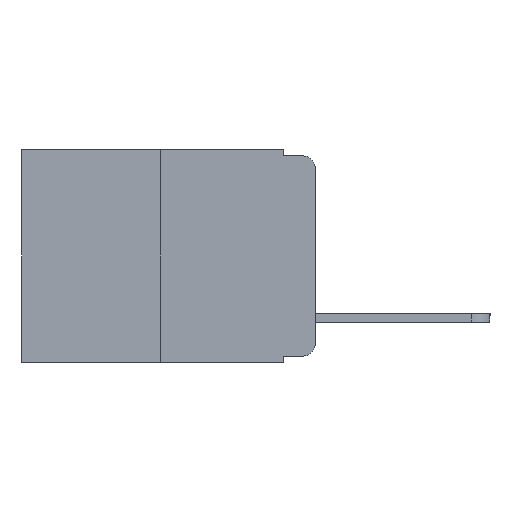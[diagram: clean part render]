
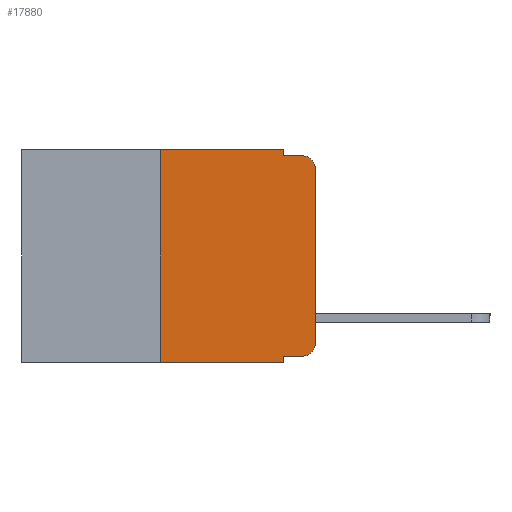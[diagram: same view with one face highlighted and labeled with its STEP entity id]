
A CAD part, left-side view. The second image highlights one B-rep face of the part: STEP entity #17880.
In plain terms, the highlighted planar face has unit normal (-1, 0, 0).
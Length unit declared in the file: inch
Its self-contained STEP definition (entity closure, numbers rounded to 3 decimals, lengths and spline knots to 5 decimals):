
#345 = EDGE_CURVE ( 'NONE', #1542, #9815, #5355, .T. ) ;
#1218 = CARTESIAN_POINT ( 'NONE',  ( 0., 0.02, -0.03 ) ) ;
#1253 = VECTOR ( 'NONE', #8142, 39.37008 ) ;
#1542 = VERTEX_POINT ( 'NONE', #8041 ) ;
#1605 = LINE ( 'NONE', #11146, #16350 ) ;
#2060 = CARTESIAN_POINT ( 'NONE',  ( 0., 0.051, 0. ) ) ;
#2106 = AXIS2_PLACEMENT_3D ( 'NONE', #1218, #11420, #2782 ) ;
#2268 = ORIENTED_EDGE ( 'NONE', *, *, #15276, .F. ) ;
#2299 = DIRECTION ( 'NONE',  ( 1., 0., 0. ) ) ;
#2311 = ORIENTED_EDGE ( 'NONE', *, *, #17517, .F. ) ;
#2459 = ORIENTED_EDGE ( 'NONE', *, *, #16205, .F. ) ;
#2679 = VECTOR ( 'NONE', #14028, 39.37008 ) ;
#2782 = DIRECTION ( 'NONE',  ( 0., 0., -1. ) ) ;
#2800 = ORIENTED_EDGE ( 'NONE', *, *, #17160, .F. ) ;
#2856 = CARTESIAN_POINT ( 'NONE',  ( 0., 0.051, -0.343 ) ) ;
#3518 = VECTOR ( 'NONE', #6257, 39.37008 ) ;
#3520 = VERTEX_POINT ( 'NONE', #3736 ) ;
#3658 = DIRECTION ( 'NONE',  ( 0., 0., -1. ) ) ;
#3736 = CARTESIAN_POINT ( 'NONE',  ( 0., 0.02, -0.01 ) ) ;
#4001 = CARTESIAN_POINT ( 'NONE',  ( 0., 0., 0. ) ) ;
#4339 = VERTEX_POINT ( 'NONE', #2856 ) ;
#4696 = AXIS2_PLACEMENT_3D ( 'NONE', #4937, #14725, #6358 ) ;
#4819 = CARTESIAN_POINT ( 'NONE',  ( 0., 0.25, 0. ) ) ;
#4910 = VECTOR ( 'NONE', #3658, 39.37008 ) ;
#4937 = CARTESIAN_POINT ( 'NONE',  ( 0., 0.02, -0.313 ) ) ;
#5074 = EDGE_LOOP ( 'NONE', ( #12669, #11623, #2800, #2459, #2311, #2268, #10667, #10511, #12202, #16881 ) ) ;
#5111 = CARTESIAN_POINT ( 'NONE',  ( 0., 0.473, -0.343 ) ) ;
#5220 = LINE ( 'NONE', #5350, #12689 ) ;
#5350 = CARTESIAN_POINT ( 'NONE',  ( 0., 0.051, -0.333 ) ) ;
#5355 = LINE ( 'NONE', #4001, #1253 ) ;
#5540 = LINE ( 'NONE', #14225, #15814 ) ;
#5560 = EDGE_CURVE ( 'NONE', #10413, #4339, #9112, .T. ) ;
#6257 = DIRECTION ( 'NONE',  ( 0., 0., 1. ) ) ;
#6358 = DIRECTION ( 'NONE',  ( 0., 0., -1. ) ) ;
#7493 = AXIS2_PLACEMENT_3D ( 'NONE', #7959, #2299, #12383 ) ;
#7753 = CARTESIAN_POINT ( 'NONE',  ( 0., 0.25, -0.343 ) ) ;
#7959 = CARTESIAN_POINT ( 'NONE',  ( 0., 0.473, 0. ) ) ;
#8041 = CARTESIAN_POINT ( 'NONE',  ( 0., 0., -0.313 ) ) ;
#8142 = DIRECTION ( 'NONE',  ( 0., 0., 1. ) ) ;
#8289 = CARTESIAN_POINT ( 'NONE',  ( 0., 0.02, -0.333 ) ) ;
#9112 = LINE ( 'NONE', #5111, #16481 ) ;
#9815 = VERTEX_POINT ( 'NONE', #14805 ) ;
#10374 = LINE ( 'NONE', #12626, #2679 ) ;
#10413 = VERTEX_POINT ( 'NONE', #7753 ) ;
#10511 = ORIENTED_EDGE ( 'NONE', *, *, #14356, .F. ) ;
#10667 = ORIENTED_EDGE ( 'NONE', *, *, #5560, .T. ) ;
#10995 = PLANE ( 'NONE',  #7493 ) ;
#11122 = LINE ( 'NONE', #4819, #3518 ) ;
#11146 = CARTESIAN_POINT ( 'NONE',  ( 0., 0.051, 0. ) ) ;
#11420 = DIRECTION ( 'NONE',  ( -1., 0., 0. ) ) ;
#11463 = VERTEX_POINT ( 'NONE', #8289 ) ;
#11623 = ORIENTED_EDGE ( 'NONE', *, *, #18081, .T. ) ;
#11999 = CARTESIAN_POINT ( 'NONE',  ( 0., 0.051, -0.01 ) ) ;
#12111 = DIRECTION ( 'NONE',  ( 0., -1., 0. ) ) ;
#12202 = ORIENTED_EDGE ( 'NONE', *, *, #13430, .T. ) ;
#12376 = LINE ( 'NONE', #2060, #4910 ) ;
#12383 = DIRECTION ( 'NONE',  ( 0., 0., -1. ) ) ;
#12479 = EDGE_CURVE ( 'NONE', #11463, #1542, #17940, .T. ) ;
#12626 = CARTESIAN_POINT ( 'NONE',  ( 0., 0.051, -0.01 ) ) ;
#12669 = ORIENTED_EDGE ( 'NONE', *, *, #345, .T. ) ;
#12689 = VECTOR ( 'NONE', #16534, 39.37008 ) ;
#13430 = EDGE_CURVE ( 'NONE', #17615, #11463, #5220, .T. ) ;
#13931 = DIRECTION ( 'NONE',  ( 0., 0., -1. ) ) ;
#14028 = DIRECTION ( 'NONE',  ( 0., -1., 0. ) ) ;
#14225 = CARTESIAN_POINT ( 'NONE',  ( 0., 0.473, 0. ) ) ;
#14356 = EDGE_CURVE ( 'NONE', #17615, #4339, #1605, .T. ) ;
#14725 = DIRECTION ( 'NONE',  ( -1., 0., 0. ) ) ;
#14805 = CARTESIAN_POINT ( 'NONE',  ( 0., 0., -0.03 ) ) ;
#14841 = VERTEX_POINT ( 'NONE', #17865 ) ;
#15120 = CARTESIAN_POINT ( 'NONE',  ( 0., 0.25, 0. ) ) ;
#15276 = EDGE_CURVE ( 'NONE', #10413, #16991, #11122, .T. ) ;
#15795 = CIRCLE ( 'NONE', #2106, 0.02 ) ;
#15814 = VECTOR ( 'NONE', #17030, 39.37008 ) ;
#16128 = VERTEX_POINT ( 'NONE', #11999 ) ;
#16205 = EDGE_CURVE ( 'NONE', #14841, #16128, #12376, .T. ) ;
#16350 = VECTOR ( 'NONE', #13931, 39.37008 ) ;
#16481 = VECTOR ( 'NONE', #12111, 39.37008 ) ;
#16534 = DIRECTION ( 'NONE',  ( 0., -1., 0. ) ) ;
#16881 = ORIENTED_EDGE ( 'NONE', *, *, #12479, .T. ) ;
#16991 = VERTEX_POINT ( 'NONE', #15120 ) ;
#17030 = DIRECTION ( 'NONE',  ( 0., -1., 0. ) ) ;
#17160 = EDGE_CURVE ( 'NONE', #16128, #3520, #10374, .T. ) ;
#17219 = CARTESIAN_POINT ( 'NONE',  ( 0., 0.051, -0.333 ) ) ;
#17517 = EDGE_CURVE ( 'NONE', #16991, #14841, #5540, .T. ) ;
#17615 = VERTEX_POINT ( 'NONE', #17219 ) ;
#17865 = CARTESIAN_POINT ( 'NONE',  ( 0., 0.051, 0. ) ) ;
#17880 = ADVANCED_FACE ( 'NONE', ( #17979 ), #10995, .F. ) ;
#17940 = CIRCLE ( 'NONE', #4696, 0.02 ) ;
#17979 = FACE_OUTER_BOUND ( 'NONE', #5074, .T. ) ;
#18081 = EDGE_CURVE ( 'NONE', #9815, #3520, #15795, .T. ) ;
